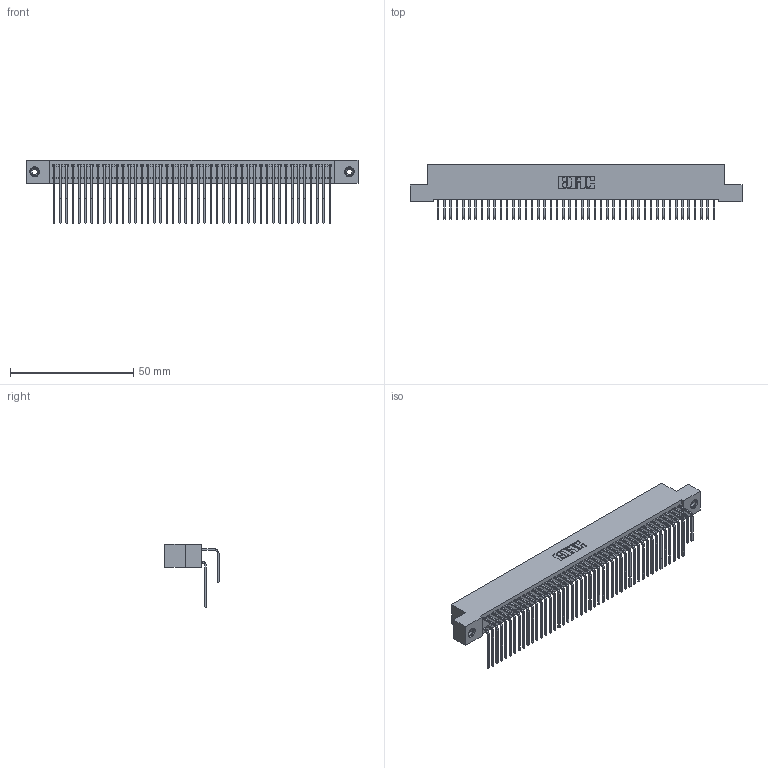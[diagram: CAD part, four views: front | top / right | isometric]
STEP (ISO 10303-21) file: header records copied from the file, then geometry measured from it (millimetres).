
FILE_DESCRIPTION (( 'STEP AP203' ), '1' );
FILE_NAME ('392-090-558-208.STEP', '2019-10-09T18:38:08', ( '' ), ( '' ), 'SwSTEP 2.0', 'SolidWorks 2016', '' );
FILE_SCHEMA (( 'CONFIG_CONTROL_DESIGN' ));
Length unit declared in the file: inch
Products named in the file (5): 345-250-001_345-250-003-102; 392-090-558-208; 342 Part_TI; 345-292-001_558 559 Tail - 1; 345-292-001_558 Tail - 2
Assembly tree (93 placements, depth 2):
  392-090-558-208
    342 Part_TI
    345-292-001_558 559 Tail - 1  x45
    345-292-001_558 Tail - 2  x45
    345-250-001_345-250-003-102  x2
Bounding box: 134.62 x 21.91 x 25.78 mm (x, y, z)
Volume: 12623.3 mm3; surface area: 22980.4 mm2
Topology: 93 solids, 93 shells, 5030 faces, 14925 edges, 9822 vertices
Faces by surface type: plane 3518, cylinder 1496, cone 12, torus 4
Entity records: 31400 total; most frequent: CARTESIAN_POINT 5232, ORIENTED_EDGE 5110, DIRECTION 4477, EDGE_CURVE 2555, VECTOR 2367, LINE 2367, VERTEX_POINT 1696, AXIS2_PLACEMENT_3D 1055
